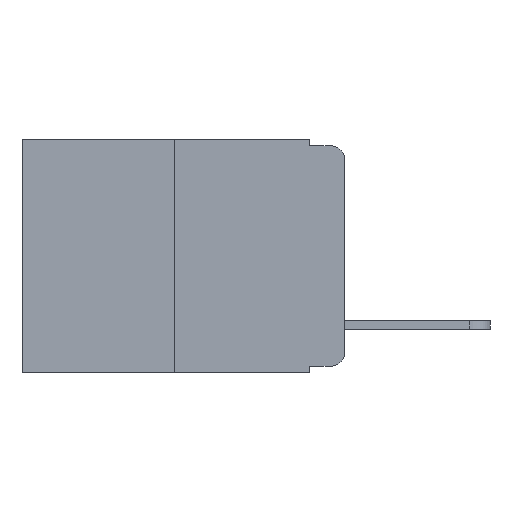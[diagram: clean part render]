
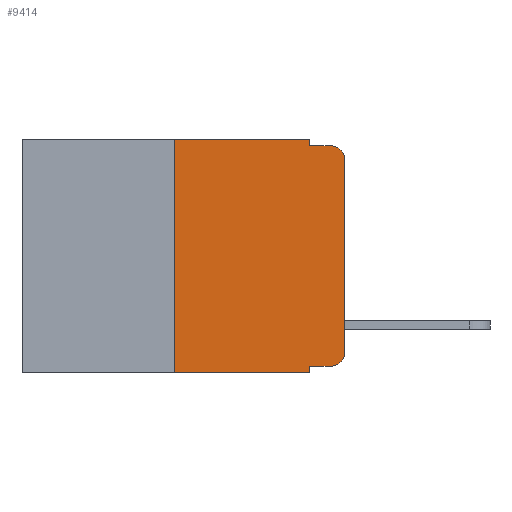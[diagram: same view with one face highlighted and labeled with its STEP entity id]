
A CAD part, left-side view. The second image highlights one B-rep face of the part: STEP entity #9414.
In plain terms, the highlighted planar face has unit normal (-1, 0, 0).
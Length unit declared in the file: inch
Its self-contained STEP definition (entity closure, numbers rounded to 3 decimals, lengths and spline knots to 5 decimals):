
#36 = CARTESIAN_POINT ( 'NONE',  ( 0., 0.02, -0.333 ) ) ;
#78 = EDGE_CURVE ( 'NONE', #18414, #10039, #5323, .T. ) ;
#482 = ORIENTED_EDGE ( 'NONE', *, *, #6272, .T. ) ;
#640 = VERTEX_POINT ( 'NONE', #7482 ) ;
#797 = VECTOR ( 'NONE', #3430, 39.37008 ) ;
#939 = VERTEX_POINT ( 'NONE', #11949 ) ;
#955 = VERTEX_POINT ( 'NONE', #4156 ) ;
#1236 = CARTESIAN_POINT ( 'NONE',  ( 0., 0.25, -0.343 ) ) ;
#1391 = VECTOR ( 'NONE', #19089, 39.37008 ) ;
#2066 = LINE ( 'NONE', #17026, #9247 ) ;
#2265 = CARTESIAN_POINT ( 'NONE',  ( 0., 0.051, -0.333 ) ) ;
#2571 = ORIENTED_EDGE ( 'NONE', *, *, #10599, .T. ) ;
#3200 = CARTESIAN_POINT ( 'NONE',  ( 0., 0.473, 0. ) ) ;
#3430 = DIRECTION ( 'NONE',  ( 0., -1., 0. ) ) ;
#4073 = VECTOR ( 'NONE', #19246, 39.37008 ) ;
#4156 = CARTESIAN_POINT ( 'NONE',  ( 0., 0., -0.313 ) ) ;
#4206 = DIRECTION ( 'NONE',  ( 0., -1., 0. ) ) ;
#4276 = CIRCLE ( 'NONE', #21131, 0.02 ) ;
#4323 = LINE ( 'NONE', #10671, #4073 ) ;
#4444 = EDGE_CURVE ( 'NONE', #12472, #10039, #15744, .T. ) ;
#4803 = DIRECTION ( 'NONE',  ( 0., 0., -1. ) ) ;
#5323 = LINE ( 'NONE', #6687, #797 ) ;
#5413 = VERTEX_POINT ( 'NONE', #15929 ) ;
#6033 = EDGE_CURVE ( 'NONE', #640, #939, #2066, .T. ) ;
#6051 = DIRECTION ( 'NONE',  ( -1., 0., 0. ) ) ;
#6272 = EDGE_CURVE ( 'NONE', #955, #16096, #13279, .T. ) ;
#6547 = DIRECTION ( 'NONE',  ( 0., -1., 0. ) ) ;
#6683 = DIRECTION ( 'NONE',  ( 0., 0., -1. ) ) ;
#6687 = CARTESIAN_POINT ( 'NONE',  ( 0., 0.473, -0.343 ) ) ;
#6841 = LINE ( 'NONE', #13281, #10858 ) ;
#7007 = DIRECTION ( 'NONE',  ( 0., -1., 0. ) ) ;
#7100 = VECTOR ( 'NONE', #9440, 39.37008 ) ;
#7482 = CARTESIAN_POINT ( 'NONE',  ( 0., 0.051, -0.01 ) ) ;
#7708 = ORIENTED_EDGE ( 'NONE', *, *, #12648, .T. ) ;
#7837 = CARTESIAN_POINT ( 'NONE',  ( 0., 0.02, -0.313 ) ) ;
#8261 = ORIENTED_EDGE ( 'NONE', *, *, #78, .T. ) ;
#8392 = DIRECTION ( 'NONE',  ( 1., 0., 0. ) ) ;
#9129 = EDGE_CURVE ( 'NONE', #5413, #640, #9358, .T. ) ;
#9247 = VECTOR ( 'NONE', #7007, 39.37008 ) ;
#9358 = LINE ( 'NONE', #12388, #1391 ) ;
#9397 = CARTESIAN_POINT ( 'NONE',  ( 0., 0.25, 0. ) ) ;
#9414 = ADVANCED_FACE ( 'NONE', ( #15048 ), #9897, .F. ) ;
#9440 = DIRECTION ( 'NONE',  ( 0., 0., 1. ) ) ;
#9700 = EDGE_CURVE ( 'NONE', #18414, #21497, #4323, .T. ) ;
#9710 = DIRECTION ( 'NONE',  ( 0., 0., -1. ) ) ;
#9897 = PLANE ( 'NONE',  #18087 ) ;
#9929 = ORIENTED_EDGE ( 'NONE', *, *, #19764, .T. ) ;
#10039 = VERTEX_POINT ( 'NONE', #11940 ) ;
#10599 = EDGE_CURVE ( 'NONE', #16096, #939, #4276, .T. ) ;
#10600 = ORIENTED_EDGE ( 'NONE', *, *, #6033, .F. ) ;
#10671 = CARTESIAN_POINT ( 'NONE',  ( 0., 0.25, 0. ) ) ;
#10858 = VECTOR ( 'NONE', #6547, 39.37008 ) ;
#11288 = EDGE_CURVE ( 'NONE', #21497, #5413, #18406, .T. ) ;
#11439 = ORIENTED_EDGE ( 'NONE', *, *, #9129, .F. ) ;
#11615 = VERTEX_POINT ( 'NONE', #36 ) ;
#11940 = CARTESIAN_POINT ( 'NONE',  ( 0., 0.051, -0.343 ) ) ;
#11949 = CARTESIAN_POINT ( 'NONE',  ( 0., 0.02, -0.01 ) ) ;
#12388 = CARTESIAN_POINT ( 'NONE',  ( 0., 0.051, 0. ) ) ;
#12472 = VERTEX_POINT ( 'NONE', #2265 ) ;
#12648 = EDGE_CURVE ( 'NONE', #11615, #955, #18337, .T. ) ;
#13279 = LINE ( 'NONE', #19687, #7100 ) ;
#13281 = CARTESIAN_POINT ( 'NONE',  ( 0., 0.051, -0.333 ) ) ;
#14236 = ORIENTED_EDGE ( 'NONE', *, *, #11288, .F. ) ;
#14406 = VECTOR ( 'NONE', #4206, 39.37008 ) ;
#14550 = CARTESIAN_POINT ( 'NONE',  ( 0., 0.051, 0. ) ) ;
#14730 = AXIS2_PLACEMENT_3D ( 'NONE', #7837, #6051, #9710 ) ;
#14891 = DIRECTION ( 'NONE',  ( -1., 0., 0. ) ) ;
#15048 = FACE_OUTER_BOUND ( 'NONE', #15369, .T. ) ;
#15369 = EDGE_LOOP ( 'NONE', ( #482, #2571, #10600, #11439, #14236, #20614, #8261, #17045, #9929, #7708 ) ) ;
#15744 = LINE ( 'NONE', #14550, #21370 ) ;
#15929 = CARTESIAN_POINT ( 'NONE',  ( 0., 0.051, 0. ) ) ;
#16096 = VERTEX_POINT ( 'NONE', #22080 ) ;
#16275 = DIRECTION ( 'NONE',  ( 0., 0., -1. ) ) ;
#16600 = CARTESIAN_POINT ( 'NONE',  ( 0., 0.02, -0.03 ) ) ;
#17026 = CARTESIAN_POINT ( 'NONE',  ( 0., 0.051, -0.01 ) ) ;
#17045 = ORIENTED_EDGE ( 'NONE', *, *, #4444, .F. ) ;
#18087 = AXIS2_PLACEMENT_3D ( 'NONE', #3200, #8392, #6683 ) ;
#18337 = CIRCLE ( 'NONE', #14730, 0.02 ) ;
#18406 = LINE ( 'NONE', #19422, #14406 ) ;
#18414 = VERTEX_POINT ( 'NONE', #1236 ) ;
#19089 = DIRECTION ( 'NONE',  ( 0., 0., -1. ) ) ;
#19246 = DIRECTION ( 'NONE',  ( 0., 0., 1. ) ) ;
#19422 = CARTESIAN_POINT ( 'NONE',  ( 0., 0.473, 0. ) ) ;
#19687 = CARTESIAN_POINT ( 'NONE',  ( 0., 0., 0. ) ) ;
#19764 = EDGE_CURVE ( 'NONE', #12472, #11615, #6841, .T. ) ;
#20614 = ORIENTED_EDGE ( 'NONE', *, *, #9700, .F. ) ;
#21131 = AXIS2_PLACEMENT_3D ( 'NONE', #16600, #14891, #4803 ) ;
#21370 = VECTOR ( 'NONE', #16275, 39.37008 ) ;
#21497 = VERTEX_POINT ( 'NONE', #9397 ) ;
#22080 = CARTESIAN_POINT ( 'NONE',  ( 0., 0., -0.03 ) ) ;
